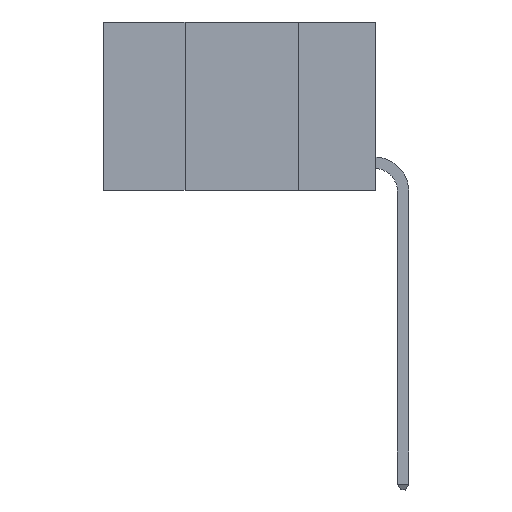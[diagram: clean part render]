
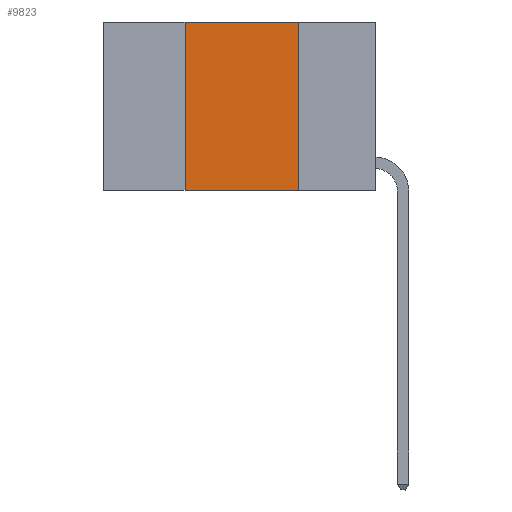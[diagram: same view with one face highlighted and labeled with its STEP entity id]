
A CAD part, left-side view. The second image highlights one B-rep face of the part: STEP entity #9823.
In plain terms, the highlighted planar face has unit normal (-1, 0, 0).
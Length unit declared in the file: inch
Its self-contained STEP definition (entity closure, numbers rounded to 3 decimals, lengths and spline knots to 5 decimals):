
#180 = VERTEX_POINT ( 'NONE', #1490 ) ;
#433 = CARTESIAN_POINT ( 'NONE',  ( 0., 0.6, -0.37 ) ) ;
#530 = DIRECTION ( 'NONE',  ( 0., 0., -1. ) ) ;
#729 = DIRECTION ( 'NONE',  ( 0., 0., -1. ) ) ;
#860 = FACE_OUTER_BOUND ( 'NONE', #6344, .T. ) ;
#1031 = CARTESIAN_POINT ( 'NONE',  ( 0., 0.42, 0. ) ) ;
#1253 = DIRECTION ( 'NONE',  ( 0., -1., 0. ) ) ;
#1490 = CARTESIAN_POINT ( 'NONE',  ( 0., 0.17, 0. ) ) ;
#2418 = ORIENTED_EDGE ( 'NONE', *, *, #5390, .F. ) ;
#2706 = ORIENTED_EDGE ( 'NONE', *, *, #4684, .T. ) ;
#2744 = VERTEX_POINT ( 'NONE', #8545 ) ;
#3960 = PLANE ( 'NONE',  #5434 ) ;
#4065 = ORIENTED_EDGE ( 'NONE', *, *, #5195, .F. ) ;
#4271 = DIRECTION ( 'NONE',  ( 0., 0., 1. ) ) ;
#4577 = VECTOR ( 'NONE', #4271, 39.37008 ) ;
#4684 = EDGE_CURVE ( 'NONE', #8718, #2744, #7521, .T. ) ;
#4816 = CARTESIAN_POINT ( 'NONE',  ( 0., 0.6, 0. ) ) ;
#4942 = LINE ( 'NONE', #4816, #8675 ) ;
#5009 = EDGE_CURVE ( 'NONE', #6898, #180, #4942, .T. ) ;
#5083 = CARTESIAN_POINT ( 'NONE',  ( 0., 0.42, -0.37 ) ) ;
#5195 = EDGE_CURVE ( 'NONE', #8718, #6898, #6653, .T. ) ;
#5390 = EDGE_CURVE ( 'NONE', #180, #2744, #6762, .T. ) ;
#5415 = VECTOR ( 'NONE', #1253, 39.37008 ) ;
#5434 = AXIS2_PLACEMENT_3D ( 'NONE', #9428, #5515, #729 ) ;
#5515 = DIRECTION ( 'NONE',  ( 1., 0., 0. ) ) ;
#6344 = EDGE_LOOP ( 'NONE', ( #2418, #8701, #4065, #2706 ) ) ;
#6653 = LINE ( 'NONE', #1031, #4577 ) ;
#6762 = LINE ( 'NONE', #9228, #8669 ) ;
#6898 = VERTEX_POINT ( 'NONE', #8392 ) ;
#7521 = LINE ( 'NONE', #433, #5415 ) ;
#8392 = CARTESIAN_POINT ( 'NONE',  ( 0., 0.42, 0. ) ) ;
#8545 = CARTESIAN_POINT ( 'NONE',  ( 0., 0.17, -0.37 ) ) ;
#8669 = VECTOR ( 'NONE', #530, 39.37008 ) ;
#8675 = VECTOR ( 'NONE', #9509, 39.37008 ) ;
#8701 = ORIENTED_EDGE ( 'NONE', *, *, #5009, .F. ) ;
#8718 = VERTEX_POINT ( 'NONE', #5083 ) ;
#9228 = CARTESIAN_POINT ( 'NONE',  ( 0., 0.17, 0. ) ) ;
#9428 = CARTESIAN_POINT ( 'NONE',  ( 0., 0.6, 0. ) ) ;
#9509 = DIRECTION ( 'NONE',  ( 0., -1., 0. ) ) ;
#9823 = ADVANCED_FACE ( 'NONE', ( #860 ), #3960, .F. ) ;
